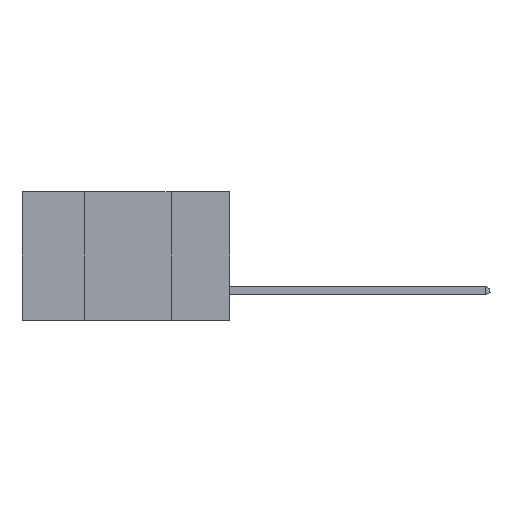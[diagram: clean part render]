
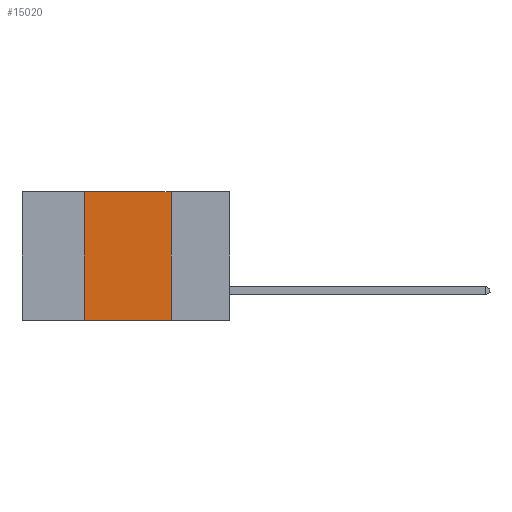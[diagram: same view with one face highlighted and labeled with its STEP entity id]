
A CAD part, left-side view. The second image highlights one B-rep face of the part: STEP entity #15020.
In plain terms, the highlighted planar face has unit normal (-1, 0, 0).
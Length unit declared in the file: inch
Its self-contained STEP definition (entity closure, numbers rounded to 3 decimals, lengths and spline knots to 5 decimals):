
#1005 = PLANE ( 'NONE',  #17554 ) ;
#1803 = ORIENTED_EDGE ( 'NONE', *, *, #12744, .F. ) ;
#2176 = VERTEX_POINT ( 'NONE', #13735 ) ;
#2468 = ORIENTED_EDGE ( 'NONE', *, *, #4257, .T. ) ;
#4006 = DIRECTION ( 'NONE',  ( 0., -1., 0. ) ) ;
#4257 = EDGE_CURVE ( 'NONE', #2176, #6007, #13956, .T. ) ;
#4697 = ORIENTED_EDGE ( 'NONE', *, *, #11540, .F. ) ;
#4892 = VECTOR ( 'NONE', #12797, 39.37008 ) ;
#5349 = CARTESIAN_POINT ( 'NONE',  ( 0., 0.17, 0. ) ) ;
#5978 = CARTESIAN_POINT ( 'NONE',  ( 0., 0.42, 0. ) ) ;
#6007 = VERTEX_POINT ( 'NONE', #17333 ) ;
#7482 = CARTESIAN_POINT ( 'NONE',  ( 0., 0.17, 0. ) ) ;
#10266 = EDGE_LOOP ( 'NONE', ( #12536, #1803, #4697, #2468 ) ) ;
#10675 = EDGE_CURVE ( 'NONE', #18510, #6007, #21685, .T. ) ;
#10946 = VECTOR ( 'NONE', #4006, 39.37008 ) ;
#11342 = LINE ( 'NONE', #5978, #23177 ) ;
#11459 = DIRECTION ( 'NONE',  ( 0., 0., -1. ) ) ;
#11540 = EDGE_CURVE ( 'NONE', #2176, #18418, #11342, .T. ) ;
#12536 = ORIENTED_EDGE ( 'NONE', *, *, #10675, .F. ) ;
#12744 = EDGE_CURVE ( 'NONE', #18418, #18510, #24713, .T. ) ;
#12797 = DIRECTION ( 'NONE',  ( 0., -1., 0. ) ) ;
#13735 = CARTESIAN_POINT ( 'NONE',  ( 0., 0.42, -0.37 ) ) ;
#13956 = LINE ( 'NONE', #21063, #4892 ) ;
#15020 = ADVANCED_FACE ( 'NONE', ( #15288 ), #1005, .F. ) ;
#15288 = FACE_OUTER_BOUND ( 'NONE', #10266, .T. ) ;
#15765 = VECTOR ( 'NONE', #21272, 39.37008 ) ;
#16981 = CARTESIAN_POINT ( 'NONE',  ( 0., 0.6, 0. ) ) ;
#17333 = CARTESIAN_POINT ( 'NONE',  ( 0., 0.17, -0.37 ) ) ;
#17484 = CARTESIAN_POINT ( 'NONE',  ( 0., 0.42, 0. ) ) ;
#17554 = AXIS2_PLACEMENT_3D ( 'NONE', #16981, #18940, #11459 ) ;
#18418 = VERTEX_POINT ( 'NONE', #17484 ) ;
#18510 = VERTEX_POINT ( 'NONE', #7482 ) ;
#18940 = DIRECTION ( 'NONE',  ( 1., 0., 0. ) ) ;
#19907 = DIRECTION ( 'NONE',  ( 0., 0., 1. ) ) ;
#21063 = CARTESIAN_POINT ( 'NONE',  ( 0., 0.6, -0.37 ) ) ;
#21272 = DIRECTION ( 'NONE',  ( 0., 0., -1. ) ) ;
#21685 = LINE ( 'NONE', #5349, #15765 ) ;
#23177 = VECTOR ( 'NONE', #19907, 39.37008 ) ;
#24146 = CARTESIAN_POINT ( 'NONE',  ( 0., 0.6, 0. ) ) ;
#24713 = LINE ( 'NONE', #24146, #10946 ) ;
